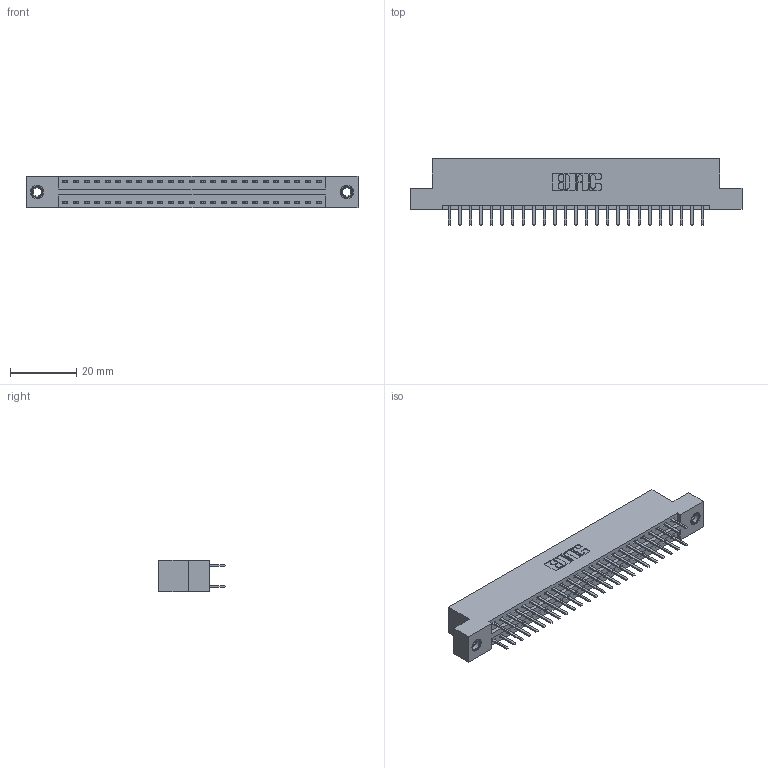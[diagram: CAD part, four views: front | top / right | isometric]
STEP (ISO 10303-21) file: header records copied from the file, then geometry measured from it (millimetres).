
FILE_DESCRIPTION (( 'STEP AP203' ), '1' );
FILE_NAME ('396-050-520-207.STEP', '2018-09-08T02:53:27', ( '' ), ( '' ), 'SwSTEP 2.0', 'SolidWorks 2016', '' );
FILE_SCHEMA (( 'CONFIG_CONTROL_DESIGN' ));
Length unit declared in the file: inch
Products named in the file (4): 345-250-001_345-250-005-103; 396-050-520-207; 346 Part_Flush Mounting Lugs - 0.156 Dia-TI; 345-292-001_345-293-120
Assembly tree (53 placements, depth 2):
  396-050-520-207
    346 Part_Flush Mounting Lugs - 0.156 Dia-TI
    345-292-001_345-293-120  x50
    345-250-001_345-250-005-103  x2
Bounding box: 99.95 x 20.02 x 9.4 mm (x, y, z)
Volume: 9578.7 mm3; surface area: 12881.7 mm2
Topology: 53 solids, 53 shells, 2982 faces, 8615 edges, 5602 vertices
Faces by surface type: plane 1958, cylinder 1008, cone 12, torus 4
Entity records: 19904 total; most frequent: CARTESIAN_POINT 3299, ORIENTED_EDGE 3214, DIRECTION 2973, EDGE_CURVE 1607, VECTOR 1351, LINE 1351, VERTEX_POINT 1064, AXIS2_PLACEMENT_3D 811
